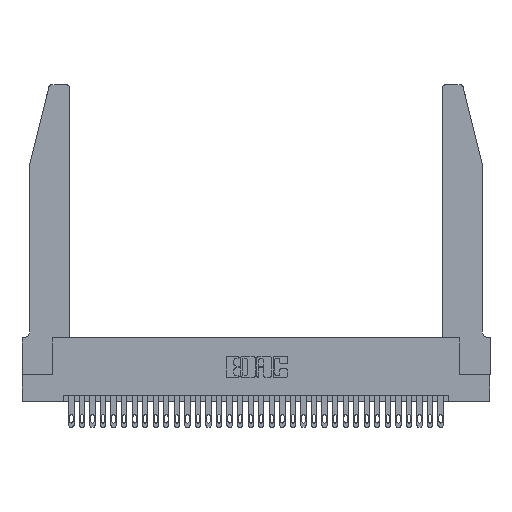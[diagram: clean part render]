
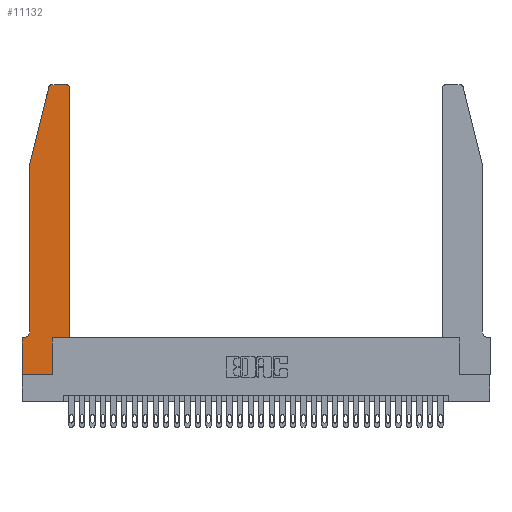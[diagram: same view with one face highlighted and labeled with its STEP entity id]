
A CAD part, top view. The second image highlights one B-rep face of the part: STEP entity #11132.
In plain terms, the highlighted planar face has unit normal (0, 0, 1).
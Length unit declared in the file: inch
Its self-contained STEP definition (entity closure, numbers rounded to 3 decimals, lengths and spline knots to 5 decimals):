
#54 = CIRCLE ( 'NONE', #20157, 0.03 ) ;
#530 = DIRECTION ( 'NONE',  ( 0., 0., 1. ) ) ;
#624 = DIRECTION ( 'NONE',  ( 0., -1., 0. ) ) ;
#870 = VECTOR ( 'NONE', #16085, 39.37008 ) ;
#1623 = LINE ( 'NONE', #25182, #32202 ) ;
#1728 = EDGE_CURVE ( 'NONE', #5067, #6898, #27029, .T. ) ;
#1931 = ORIENTED_EDGE ( 'NONE', *, *, #24392, .T. ) ;
#2490 = VECTOR ( 'NONE', #18636, 39.37008 ) ;
#2632 = EDGE_CURVE ( 'NONE', #8499, #18519, #19456, .T. ) ;
#2847 = DIRECTION ( 'NONE',  ( 0., 1., 0. ) ) ;
#2996 = VECTOR ( 'NONE', #24645, 39.37008 ) ;
#3602 = ORIENTED_EDGE ( 'NONE', *, *, #29773, .T. ) ;
#3991 = CARTESIAN_POINT ( 'NONE',  ( 0.4505, 0.35, 0.37 ) ) ;
#4660 = VERTEX_POINT ( 'NONE', #5160 ) ;
#4764 = ORIENTED_EDGE ( 'NONE', *, *, #23475, .T. ) ;
#5067 = VERTEX_POINT ( 'NONE', #22945 ) ;
#5115 = DIRECTION ( 'NONE',  ( 0., 0., -1. ) ) ;
#5160 = CARTESIAN_POINT ( 'NONE',  ( 0.0055, 0.35, 0.37 ) ) ;
#5667 = DIRECTION ( 'NONE',  ( -1., 0., 0. ) ) ;
#5777 = CARTESIAN_POINT ( 'NONE',  ( 0.2865, 0.35, 0.37 ) ) ;
#6434 = DIRECTION ( 'NONE',  ( -0.239, -0.971, 0. ) ) ;
#6527 = CARTESIAN_POINT ( 'NONE',  ( 0.4505, 0.35, 0.37 ) ) ;
#6564 = CARTESIAN_POINT ( 'NONE',  ( 0.4205, 2.75, 0.37 ) ) ;
#6898 = VERTEX_POINT ( 'NONE', #27065 ) ;
#7243 = ORIENTED_EDGE ( 'NONE', *, *, #23885, .T. ) ;
#7419 = CARTESIAN_POINT ( 'NONE',  ( 0.0055, 0.42, 0.37 ) ) ;
#8068 = CARTESIAN_POINT ( 'NONE',  ( 0.284, 2.75, 0.37 ) ) ;
#8195 = DIRECTION ( 'NONE',  ( 1., 0., 0. ) ) ;
#8499 = VERTEX_POINT ( 'NONE', #21649 ) ;
#8673 = EDGE_CURVE ( 'NONE', #23531, #4660, #10605, .T. ) ;
#9142 = LINE ( 'NONE', #3991, #2996 ) ;
#9146 = EDGE_CURVE ( 'NONE', #30583, #23531, #1623, .T. ) ;
#9433 = LINE ( 'NONE', #21505, #2490 ) ;
#9439 = AXIS2_PLACEMENT_3D ( 'NONE', #26807, #530, #31596 ) ;
#9478 = EDGE_CURVE ( 'NONE', #18257, #18861, #13825, .T. ) ;
#10024 = CARTESIAN_POINT ( 'NONE',  ( 0.25487, 2.72718, 0.37 ) ) ;
#10605 = CIRCLE ( 'NONE', #17414, 0.07 ) ;
#10632 = ORIENTED_EDGE ( 'NONE', *, *, #30550, .T. ) ;
#11132 = ADVANCED_FACE ( 'NONE', ( #25607 ), #31203, .T. ) ;
#12394 = ORIENTED_EDGE ( 'NONE', *, *, #8673, .T. ) ;
#13562 = LINE ( 'NONE', #14420, #16463 ) ;
#13825 = LINE ( 'NONE', #5777, #16685 ) ;
#14420 = CARTESIAN_POINT ( 'NONE',  ( 0.0755, 2., 0.37 ) ) ;
#14784 = LINE ( 'NONE', #26311, #18420 ) ;
#14801 = DIRECTION ( 'NONE',  ( 0., -1., 0. ) ) ;
#14973 = DIRECTION ( 'NONE',  ( 1., 0., 0. ) ) ;
#15392 = DIRECTION ( 'NONE',  ( 1., 0., 0. ) ) ;
#15817 = DIRECTION ( 'NONE',  ( 0., 0., 1. ) ) ;
#16085 = DIRECTION ( 'NONE',  ( -1., 0., 0. ) ) ;
#16463 = VECTOR ( 'NONE', #6434, 39.37008 ) ;
#16685 = VECTOR ( 'NONE', #24023, 39.37008 ) ;
#17253 = LINE ( 'NONE', #21203, #870 ) ;
#17407 = VERTEX_POINT ( 'NONE', #10024 ) ;
#17414 = AXIS2_PLACEMENT_3D ( 'NONE', #7419, #5115, #5667 ) ;
#17464 = CARTESIAN_POINT ( 'NONE',  ( 0., 0.35, 0.37 ) ) ;
#17569 = VERTEX_POINT ( 'NONE', #8068 ) ;
#17582 = CARTESIAN_POINT ( 'NONE',  ( 0.0755, 0.42, 0.37 ) ) ;
#17686 = ORIENTED_EDGE ( 'NONE', *, *, #23062, .T. ) ;
#18246 = CARTESIAN_POINT ( 'NONE',  ( 0.4505, 0.35, 0.37 ) ) ;
#18257 = VERTEX_POINT ( 'NONE', #19918 ) ;
#18420 = VECTOR ( 'NONE', #8195, 39.37008 ) ;
#18519 = VERTEX_POINT ( 'NONE', #6564 ) ;
#18572 = CARTESIAN_POINT ( 'NONE',  ( 0., 0., 0.37 ) ) ;
#18636 = DIRECTION ( 'NONE',  ( -1., 0., 0. ) ) ;
#18759 = CARTESIAN_POINT ( 'NONE',  ( 0.2865, 0.35, 0.37 ) ) ;
#18861 = VERTEX_POINT ( 'NONE', #18759 ) ;
#19402 = AXIS2_PLACEMENT_3D ( 'NONE', #17464, #20084, #14973 ) ;
#19456 = CIRCLE ( 'NONE', #9439, 0.03 ) ;
#19885 = ORIENTED_EDGE ( 'NONE', *, *, #9478, .T. ) ;
#19918 = CARTESIAN_POINT ( 'NONE',  ( 0.2865, 0., 0.37 ) ) ;
#20084 = DIRECTION ( 'NONE',  ( 0., 0., 1. ) ) ;
#20157 = AXIS2_PLACEMENT_3D ( 'NONE', #26314, #15817, #15392 ) ;
#20174 = ORIENTED_EDGE ( 'NONE', *, *, #1728, .T. ) ;
#21203 = CARTESIAN_POINT ( 'NONE',  ( 0.0755, 0.35, 0.37 ) ) ;
#21505 = CARTESIAN_POINT ( 'NONE',  ( 0.2605, 2.75, 0.37 ) ) ;
#21649 = CARTESIAN_POINT ( 'NONE',  ( 0.4505, 2.72, 0.37 ) ) ;
#22945 = CARTESIAN_POINT ( 'NONE',  ( 0., 0.35, 0.37 ) ) ;
#23062 = EDGE_CURVE ( 'NONE', #18861, #26701, #9142, .T. ) ;
#23475 = EDGE_CURVE ( 'NONE', #17407, #30583, #13562, .T. ) ;
#23531 = VERTEX_POINT ( 'NONE', #17582 ) ;
#23885 = EDGE_CURVE ( 'NONE', #4660, #5067, #17253, .T. ) ;
#24023 = DIRECTION ( 'NONE',  ( 0., 1., 0. ) ) ;
#24291 = EDGE_CURVE ( 'NONE', #17569, #17407, #54, .T. ) ;
#24392 = EDGE_CURVE ( 'NONE', #18519, #17569, #9433, .T. ) ;
#24588 = CARTESIAN_POINT ( 'NONE',  ( 0.0755, 2., 0.37 ) ) ;
#24617 = LINE ( 'NONE', #18246, #26645 ) ;
#24645 = DIRECTION ( 'NONE',  ( 1., 0., 0. ) ) ;
#25182 = CARTESIAN_POINT ( 'NONE',  ( 0.0755, 2., 0.37 ) ) ;
#25546 = ORIENTED_EDGE ( 'NONE', *, *, #9146, .T. ) ;
#25607 = FACE_OUTER_BOUND ( 'NONE', #28640, .T. ) ;
#26311 = CARTESIAN_POINT ( 'NONE',  ( 0., 0., 0.37 ) ) ;
#26314 = CARTESIAN_POINT ( 'NONE',  ( 0.284, 2.72, 0.37 ) ) ;
#26645 = VECTOR ( 'NONE', #2847, 39.37008 ) ;
#26701 = VERTEX_POINT ( 'NONE', #6527 ) ;
#26807 = CARTESIAN_POINT ( 'NONE',  ( 0.4205, 2.72, 0.37 ) ) ;
#27029 = LINE ( 'NONE', #18572, #29055 ) ;
#27065 = CARTESIAN_POINT ( 'NONE',  ( 0., 0., 0.37 ) ) ;
#28640 = EDGE_LOOP ( 'NONE', ( #1931, #31165, #4764, #25546, #12394, #7243, #20174, #10632, #19885, #17686, #3602, #30328 ) ) ;
#29055 = VECTOR ( 'NONE', #624, 39.37008 ) ;
#29773 = EDGE_CURVE ( 'NONE', #26701, #8499, #24617, .T. ) ;
#30328 = ORIENTED_EDGE ( 'NONE', *, *, #2632, .T. ) ;
#30550 = EDGE_CURVE ( 'NONE', #6898, #18257, #14784, .T. ) ;
#30583 = VERTEX_POINT ( 'NONE', #24588 ) ;
#31165 = ORIENTED_EDGE ( 'NONE', *, *, #24291, .T. ) ;
#31203 = PLANE ( 'NONE',  #19402 ) ;
#31596 = DIRECTION ( 'NONE',  ( 1., 0., 0. ) ) ;
#32202 = VECTOR ( 'NONE', #14801, 39.37008 ) ;
